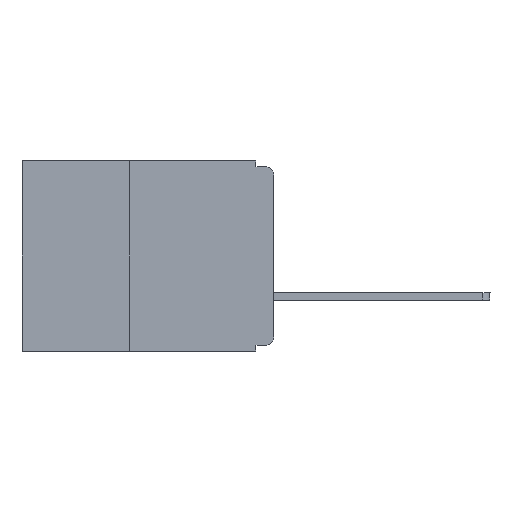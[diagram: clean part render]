
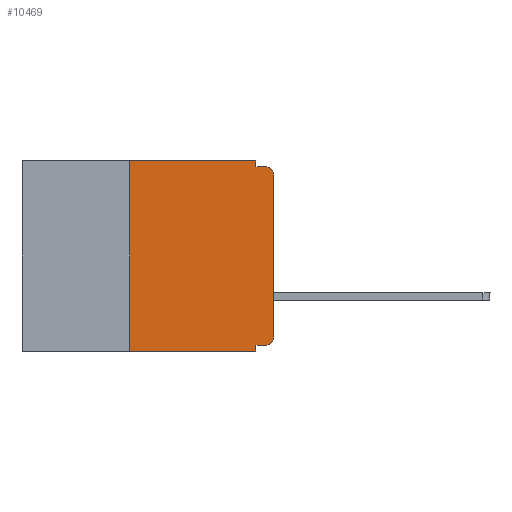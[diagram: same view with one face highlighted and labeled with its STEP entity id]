
A CAD part, left-side view. The second image highlights one B-rep face of the part: STEP entity #10469.
In plain terms, the highlighted planar face has unit normal (-1, 0, 0).
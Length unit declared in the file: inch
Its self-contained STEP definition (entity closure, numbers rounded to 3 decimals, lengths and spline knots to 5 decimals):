
#99 = ORIENTED_EDGE ( 'NONE', *, *, #4628, .F. ) ;
#277 = EDGE_LOOP ( 'NONE', ( #10695, #12487, #99, #8552, #4408, #7956, #7908, #13013, #9114, #5716 ) ) ;
#346 = VECTOR ( 'NONE', #7693, 39.37008 ) ;
#451 = EDGE_CURVE ( 'NONE', #12984, #1612, #7006, .T. ) ;
#661 = VECTOR ( 'NONE', #1712, 39.37008 ) ;
#867 = CARTESIAN_POINT ( 'NONE',  ( 0., 0., 0. ) ) ;
#971 = CIRCLE ( 'NONE', #14818, 0.015 ) ;
#983 = CARTESIAN_POINT ( 'NONE',  ( 0., 0.437, -0.33 ) ) ;
#1032 = VERTEX_POINT ( 'NONE', #12710 ) ;
#1130 = DIRECTION ( 'NONE',  ( 0., 0., 1. ) ) ;
#1361 = CARTESIAN_POINT ( 'NONE',  ( 0., 0.25, -0.33 ) ) ;
#1585 = LINE ( 'NONE', #12277, #11885 ) ;
#1612 = VERTEX_POINT ( 'NONE', #8469 ) ;
#1712 = DIRECTION ( 'NONE',  ( 0., 0., -1. ) ) ;
#1766 = DIRECTION ( 'NONE',  ( 0., 0., 1. ) ) ;
#2173 = CIRCLE ( 'NONE', #10762, 0.015 ) ;
#2365 = LINE ( 'NONE', #9213, #14311 ) ;
#2471 = LINE ( 'NONE', #7454, #661 ) ;
#2786 = AXIS2_PLACEMENT_3D ( 'NONE', #12970, #7290, #10792 ) ;
#3967 = VECTOR ( 'NONE', #4418, 39.37008 ) ;
#4290 = DIRECTION ( 'NONE',  ( -1., 0., 0. ) ) ;
#4394 = DIRECTION ( 'NONE',  ( -1., 0., 0. ) ) ;
#4408 = ORIENTED_EDGE ( 'NONE', *, *, #8559, .F. ) ;
#4418 = DIRECTION ( 'NONE',  ( 0., 1., 0. ) ) ;
#4628 = EDGE_CURVE ( 'NONE', #1612, #14295, #2365, .T. ) ;
#4964 = EDGE_CURVE ( 'NONE', #14659, #6015, #11729, .T. ) ;
#5252 = CARTESIAN_POINT ( 'NONE',  ( 0., 0., -0.025 ) ) ;
#5691 = CARTESIAN_POINT ( 'NONE',  ( 0., 0.25, -0.33 ) ) ;
#5716 = ORIENTED_EDGE ( 'NONE', *, *, #14360, .T. ) ;
#5756 = LINE ( 'NONE', #867, #7724 ) ;
#6015 = VERTEX_POINT ( 'NONE', #6341 ) ;
#6341 = CARTESIAN_POINT ( 'NONE',  ( 0., 0.25, 0. ) ) ;
#7006 = LINE ( 'NONE', #10804, #346 ) ;
#7290 = DIRECTION ( 'NONE',  ( 1., 0., 0. ) ) ;
#7454 = CARTESIAN_POINT ( 'NONE',  ( 0., 0.031, -0.33 ) ) ;
#7693 = DIRECTION ( 'NONE',  ( 0., 0., -1. ) ) ;
#7724 = VECTOR ( 'NONE', #1766, 39.37008 ) ;
#7908 = ORIENTED_EDGE ( 'NONE', *, *, #12214, .T. ) ;
#7956 = ORIENTED_EDGE ( 'NONE', *, *, #4964, .F. ) ;
#8248 = EDGE_CURVE ( 'NONE', #9553, #8614, #5756, .T. ) ;
#8469 = CARTESIAN_POINT ( 'NONE',  ( 0., 0.031, -0.01 ) ) ;
#8552 = ORIENTED_EDGE ( 'NONE', *, *, #451, .F. ) ;
#8559 = EDGE_CURVE ( 'NONE', #6015, #12984, #1585, .T. ) ;
#8614 = VERTEX_POINT ( 'NONE', #5252 ) ;
#8742 = FACE_OUTER_BOUND ( 'NONE', #277, .T. ) ;
#9046 = DIRECTION ( 'NONE',  ( 0., -1., 0. ) ) ;
#9114 = ORIENTED_EDGE ( 'NONE', *, *, #13370, .F. ) ;
#9213 = CARTESIAN_POINT ( 'NONE',  ( 0., 0., -0.01 ) ) ;
#9553 = VERTEX_POINT ( 'NONE', #11584 ) ;
#9755 = DIRECTION ( 'NONE',  ( 0., 0., -1. ) ) ;
#10469 = ADVANCED_FACE ( 'NONE', ( #8742 ), #11796, .F. ) ;
#10695 = ORIENTED_EDGE ( 'NONE', *, *, #8248, .T. ) ;
#10762 = AXIS2_PLACEMENT_3D ( 'NONE', #11033, #4394, #9755 ) ;
#10792 = DIRECTION ( 'NONE',  ( 0., 0., -1. ) ) ;
#10804 = CARTESIAN_POINT ( 'NONE',  ( 0., 0.031, 0. ) ) ;
#11033 = CARTESIAN_POINT ( 'NONE',  ( 0., 0.015, -0.305 ) ) ;
#11089 = DIRECTION ( 'NONE',  ( 0., -1., 0. ) ) ;
#11091 = CARTESIAN_POINT ( 'NONE',  ( 0., 0.015, -0.01 ) ) ;
#11325 = CARTESIAN_POINT ( 'NONE',  ( 0., 0.015, -0.025 ) ) ;
#11346 = CARTESIAN_POINT ( 'NONE',  ( 0., 0., -0.32 ) ) ;
#11377 = VECTOR ( 'NONE', #1130, 39.37008 ) ;
#11536 = EDGE_CURVE ( 'NONE', #8614, #14295, #971, .T. ) ;
#11584 = CARTESIAN_POINT ( 'NONE',  ( 0., 0., -0.305 ) ) ;
#11729 = LINE ( 'NONE', #5691, #11377 ) ;
#11796 = PLANE ( 'NONE',  #2786 ) ;
#11885 = VECTOR ( 'NONE', #11089, 39.37008 ) ;
#11902 = VERTEX_POINT ( 'NONE', #12917 ) ;
#12049 = EDGE_CURVE ( 'NONE', #11902, #12201, #2471, .T. ) ;
#12147 = LINE ( 'NONE', #983, #13255 ) ;
#12201 = VERTEX_POINT ( 'NONE', #13665 ) ;
#12214 = EDGE_CURVE ( 'NONE', #14659, #12201, #12147, .T. ) ;
#12277 = CARTESIAN_POINT ( 'NONE',  ( 0., 0.437, 0. ) ) ;
#12487 = ORIENTED_EDGE ( 'NONE', *, *, #11536, .T. ) ;
#12496 = DIRECTION ( 'NONE',  ( 0., 0., -1. ) ) ;
#12710 = CARTESIAN_POINT ( 'NONE',  ( 0., 0.015, -0.32 ) ) ;
#12837 = CARTESIAN_POINT ( 'NONE',  ( 0., 0.031, 0. ) ) ;
#12917 = CARTESIAN_POINT ( 'NONE',  ( 0., 0.031, -0.32 ) ) ;
#12970 = CARTESIAN_POINT ( 'NONE',  ( 0., 0.437, 0. ) ) ;
#12984 = VERTEX_POINT ( 'NONE', #12837 ) ;
#13013 = ORIENTED_EDGE ( 'NONE', *, *, #12049, .F. ) ;
#13255 = VECTOR ( 'NONE', #9046, 39.37008 ) ;
#13370 = EDGE_CURVE ( 'NONE', #1032, #11902, #14504, .T. ) ;
#13665 = CARTESIAN_POINT ( 'NONE',  ( 0., 0.031, -0.33 ) ) ;
#13827 = DIRECTION ( 'NONE',  ( 0., -1., 0. ) ) ;
#14295 = VERTEX_POINT ( 'NONE', #11091 ) ;
#14311 = VECTOR ( 'NONE', #13827, 39.37008 ) ;
#14360 = EDGE_CURVE ( 'NONE', #1032, #9553, #2173, .T. ) ;
#14504 = LINE ( 'NONE', #11346, #3967 ) ;
#14659 = VERTEX_POINT ( 'NONE', #1361 ) ;
#14818 = AXIS2_PLACEMENT_3D ( 'NONE', #11325, #4290, #12496 ) ;
